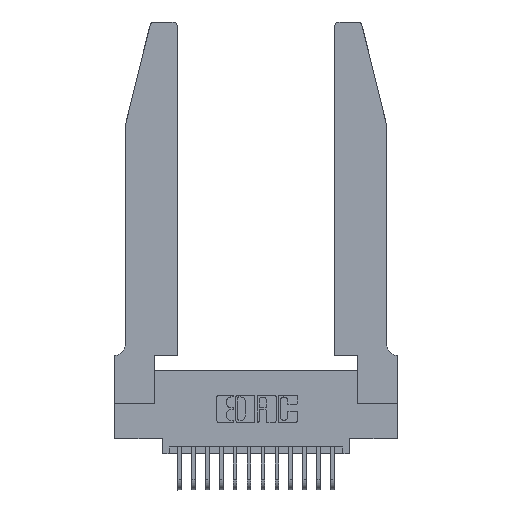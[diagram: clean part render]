
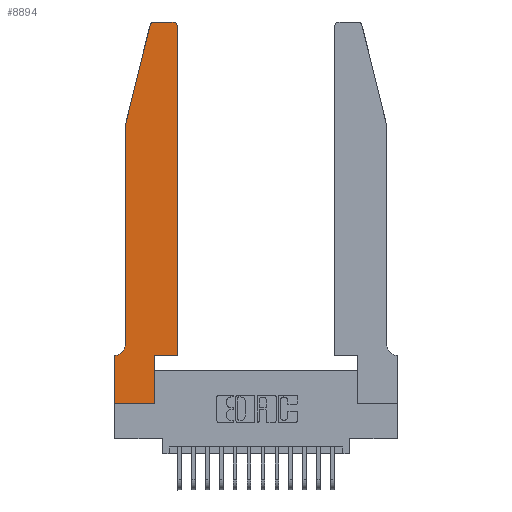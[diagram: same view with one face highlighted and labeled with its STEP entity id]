
A CAD part, top view. The second image highlights one B-rep face of the part: STEP entity #8894.
In plain terms, the highlighted planar face has unit normal (0, 0, 1).
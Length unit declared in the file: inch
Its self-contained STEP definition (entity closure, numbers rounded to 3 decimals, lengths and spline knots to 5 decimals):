
#12 = VECTOR ( 'NONE', #246, 39.37008 ) ;
#226 = CARTESIAN_POINT ( 'NONE',  ( 0.0755, 2., 0.37 ) ) ;
#246 = DIRECTION ( 'NONE',  ( 0., 1., 0. ) ) ;
#366 = VERTEX_POINT ( 'NONE', #4356 ) ;
#481 = CARTESIAN_POINT ( 'NONE',  ( 0.0755, 0.42, 0.37 ) ) ;
#526 = VERTEX_POINT ( 'NONE', #8573 ) ;
#916 = VECTOR ( 'NONE', #7702, 39.37008 ) ;
#1030 = EDGE_CURVE ( 'NONE', #8215, #16722, #13032, .T. ) ;
#1046 = AXIS2_PLACEMENT_3D ( 'NONE', #11691, #3362, #13100 ) ;
#1203 = DIRECTION ( 'NONE',  ( 0., 1., 0. ) ) ;
#1232 = ORIENTED_EDGE ( 'NONE', *, *, #9327, .T. ) ;
#1240 = DIRECTION ( 'NONE',  ( 1., 0., 0. ) ) ;
#1564 = AXIS2_PLACEMENT_3D ( 'NONE', #2744, #12497, #4159 ) ;
#1772 = DIRECTION ( 'NONE',  ( 1., 0., 0. ) ) ;
#1791 = VERTEX_POINT ( 'NONE', #12301 ) ;
#1939 = LINE ( 'NONE', #17258, #5668 ) ;
#2052 = VECTOR ( 'NONE', #1240, 39.37008 ) ;
#2104 = CARTESIAN_POINT ( 'NONE',  ( 0.0755, 2., 0.37 ) ) ;
#2338 = EDGE_CURVE ( 'NONE', #17837, #14561, #6270, .T. ) ;
#2630 = ORIENTED_EDGE ( 'NONE', *, *, #5265, .T. ) ;
#2744 = CARTESIAN_POINT ( 'NONE',  ( 0.4205, 2.72, 0.37 ) ) ;
#2915 = LINE ( 'NONE', #2104, #3363 ) ;
#3072 = CARTESIAN_POINT ( 'NONE',  ( 0.2865, 0.35, 0.37 ) ) ;
#3247 = ORIENTED_EDGE ( 'NONE', *, *, #4143, .T. ) ;
#3262 = DIRECTION ( 'NONE',  ( -0.239, -0.971, 0. ) ) ;
#3362 = DIRECTION ( 'NONE',  ( 0., 0., 1. ) ) ;
#3363 = VECTOR ( 'NONE', #6266, 39.37008 ) ;
#3383 = LINE ( 'NONE', #14597, #14047 ) ;
#3754 = EDGE_CURVE ( 'NONE', #6098, #14613, #5770, .T. ) ;
#3895 = LINE ( 'NONE', #5941, #10839 ) ;
#3944 = CIRCLE ( 'NONE', #1046, 0.03 ) ;
#4143 = EDGE_CURVE ( 'NONE', #14561, #8215, #2915, .T. ) ;
#4159 = DIRECTION ( 'NONE',  ( 1., 0., 0. ) ) ;
#4356 = CARTESIAN_POINT ( 'NONE',  ( 0.2865, 0., 0.37 ) ) ;
#4654 = LINE ( 'NONE', #9060, #916 ) ;
#4868 = ORIENTED_EDGE ( 'NONE', *, *, #14101, .T. ) ;
#5113 = CARTESIAN_POINT ( 'NONE',  ( 0., 0., 0.37 ) ) ;
#5265 = EDGE_CURVE ( 'NONE', #526, #17837, #3944, .T. ) ;
#5520 = CARTESIAN_POINT ( 'NONE',  ( 0., 0.35, 0.37 ) ) ;
#5668 = VECTOR ( 'NONE', #13136, 39.37008 ) ;
#5770 = LINE ( 'NONE', #16540, #2052 ) ;
#5941 = CARTESIAN_POINT ( 'NONE',  ( 0., 0., 0.37 ) ) ;
#6098 = VERTEX_POINT ( 'NONE', #11662 ) ;
#6100 = EDGE_CURVE ( 'NONE', #1791, #526, #1939, .T. ) ;
#6165 = ORIENTED_EDGE ( 'NONE', *, *, #14732, .T. ) ;
#6266 = DIRECTION ( 'NONE',  ( 0., -1., 0. ) ) ;
#6270 = LINE ( 'NONE', #226, #9942 ) ;
#6431 = FACE_OUTER_BOUND ( 'NONE', #16965, .T. ) ;
#6661 = EDGE_CURVE ( 'NONE', #12238, #366, #3895, .T. ) ;
#6850 = PLANE ( 'NONE',  #11597 ) ;
#6909 = DIRECTION ( 'NONE',  ( 1., 0., 0. ) ) ;
#7702 = DIRECTION ( 'NONE',  ( 0., -1., 0. ) ) ;
#8215 = VERTEX_POINT ( 'NONE', #481 ) ;
#8315 = LINE ( 'NONE', #3072, #12 ) ;
#8573 = CARTESIAN_POINT ( 'NONE',  ( 0.284, 2.75, 0.37 ) ) ;
#8642 = AXIS2_PLACEMENT_3D ( 'NONE', #15785, #15761, #15915 ) ;
#8894 = ADVANCED_FACE ( 'NONE', ( #6431 ), #6850, .T. ) ;
#9018 = DIRECTION ( 'NONE',  ( -1., 0., 0. ) ) ;
#9060 = CARTESIAN_POINT ( 'NONE',  ( 0., 0., 0.37 ) ) ;
#9139 = VERTEX_POINT ( 'NONE', #10407 ) ;
#9327 = EDGE_CURVE ( 'NONE', #14028, #1791, #14236, .T. ) ;
#9542 = CARTESIAN_POINT ( 'NONE',  ( 0.4505, 0.35, 0.37 ) ) ;
#9665 = ORIENTED_EDGE ( 'NONE', *, *, #1030, .T. ) ;
#9804 = VECTOR ( 'NONE', #1203, 39.37008 ) ;
#9942 = VECTOR ( 'NONE', #3262, 39.37008 ) ;
#10041 = CARTESIAN_POINT ( 'NONE',  ( 0.0755, 2., 0.37 ) ) ;
#10407 = CARTESIAN_POINT ( 'NONE',  ( 0., 0.35, 0.37 ) ) ;
#10490 = EDGE_CURVE ( 'NONE', #366, #6098, #8315, .T. ) ;
#10589 = ORIENTED_EDGE ( 'NONE', *, *, #2338, .T. ) ;
#10652 = ORIENTED_EDGE ( 'NONE', *, *, #16974, .T. ) ;
#10839 = VECTOR ( 'NONE', #1772, 39.37008 ) ;
#11018 = ORIENTED_EDGE ( 'NONE', *, *, #6661, .T. ) ;
#11597 = AXIS2_PLACEMENT_3D ( 'NONE', #5520, #15252, #6909 ) ;
#11662 = CARTESIAN_POINT ( 'NONE',  ( 0.2865, 0.35, 0.37 ) ) ;
#11691 = CARTESIAN_POINT ( 'NONE',  ( 0.284, 2.72, 0.37 ) ) ;
#12238 = VERTEX_POINT ( 'NONE', #5113 ) ;
#12301 = CARTESIAN_POINT ( 'NONE',  ( 0.4205, 2.75, 0.37 ) ) ;
#12497 = DIRECTION ( 'NONE',  ( 0., 0., 1. ) ) ;
#13032 = CIRCLE ( 'NONE', #8642, 0.07 ) ;
#13049 = CARTESIAN_POINT ( 'NONE',  ( 0.0055, 0.35, 0.37 ) ) ;
#13100 = DIRECTION ( 'NONE',  ( 1., 0., 0. ) ) ;
#13134 = ORIENTED_EDGE ( 'NONE', *, *, #6100, .T. ) ;
#13136 = DIRECTION ( 'NONE',  ( -1., 0., 0. ) ) ;
#13192 = ORIENTED_EDGE ( 'NONE', *, *, #3754, .T. ) ;
#14028 = VERTEX_POINT ( 'NONE', #14472 ) ;
#14047 = VECTOR ( 'NONE', #9018, 39.37008 ) ;
#14101 = EDGE_CURVE ( 'NONE', #16722, #9139, #3383, .T. ) ;
#14236 = CIRCLE ( 'NONE', #1564, 0.03 ) ;
#14386 = CARTESIAN_POINT ( 'NONE',  ( 0.4505, 0.35, 0.37 ) ) ;
#14472 = CARTESIAN_POINT ( 'NONE',  ( 0.4505, 2.72, 0.37 ) ) ;
#14561 = VERTEX_POINT ( 'NONE', #10041 ) ;
#14597 = CARTESIAN_POINT ( 'NONE',  ( 0.0755, 0.35, 0.37 ) ) ;
#14613 = VERTEX_POINT ( 'NONE', #14386 ) ;
#14732 = EDGE_CURVE ( 'NONE', #9139, #12238, #4654, .T. ) ;
#15252 = DIRECTION ( 'NONE',  ( 0., 0., 1. ) ) ;
#15761 = DIRECTION ( 'NONE',  ( 0., 0., -1. ) ) ;
#15785 = CARTESIAN_POINT ( 'NONE',  ( 0.0055, 0.42, 0.37 ) ) ;
#15915 = DIRECTION ( 'NONE',  ( -1., 0., 0. ) ) ;
#16540 = CARTESIAN_POINT ( 'NONE',  ( 0.4505, 0.35, 0.37 ) ) ;
#16682 = ORIENTED_EDGE ( 'NONE', *, *, #10490, .T. ) ;
#16722 = VERTEX_POINT ( 'NONE', #13049 ) ;
#16790 = LINE ( 'NONE', #9542, #9804 ) ;
#16965 = EDGE_LOOP ( 'NONE', ( #13134, #2630, #10589, #3247, #9665, #4868, #6165, #11018, #16682, #13192, #10652, #1232 ) ) ;
#16974 = EDGE_CURVE ( 'NONE', #14613, #14028, #16790, .T. ) ;
#17141 = CARTESIAN_POINT ( 'NONE',  ( 0.25487, 2.72718, 0.37 ) ) ;
#17258 = CARTESIAN_POINT ( 'NONE',  ( 0.2605, 2.75, 0.37 ) ) ;
#17837 = VERTEX_POINT ( 'NONE', #17141 ) ;
